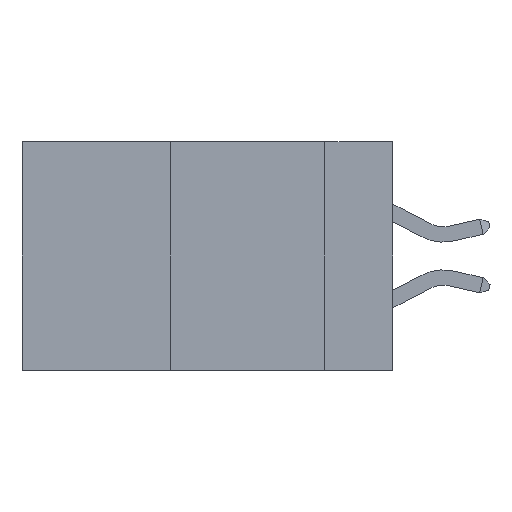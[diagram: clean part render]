
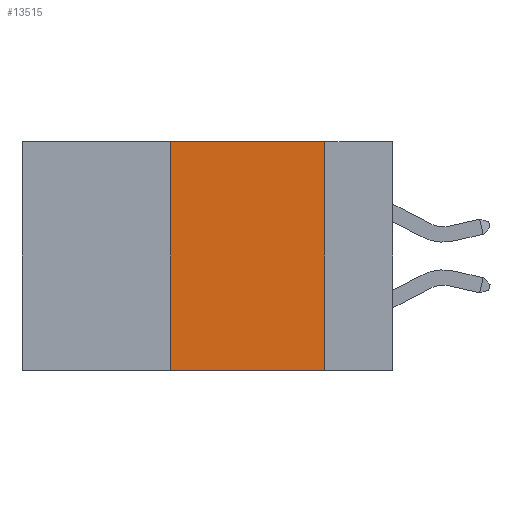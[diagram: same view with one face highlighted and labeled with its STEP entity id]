
A CAD part, left-side view. The second image highlights one B-rep face of the part: STEP entity #13515.
In plain terms, the highlighted planar face has unit normal (-1, 0, 0).
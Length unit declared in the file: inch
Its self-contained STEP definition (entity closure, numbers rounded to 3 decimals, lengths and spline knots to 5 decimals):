
#976 = ORIENTED_EDGE ( 'NONE', *, *, #16483, .F. ) ;
#1418 = LINE ( 'NONE', #15476, #12829 ) ;
#2064 = VECTOR ( 'NONE', #10358, 39.37008 ) ;
#2634 = CARTESIAN_POINT ( 'NONE',  ( 0., 0.11, -0.37 ) ) ;
#2716 = CARTESIAN_POINT ( 'NONE',  ( 0., 0.11, 0. ) ) ;
#6005 = LINE ( 'NONE', #25406, #21736 ) ;
#6934 = EDGE_CURVE ( 'NONE', #15192, #10116, #26371, .T. ) ;
#8670 = VERTEX_POINT ( 'NONE', #2716 ) ;
#9375 = CARTESIAN_POINT ( 'NONE',  ( 0., 0.36, 0. ) ) ;
#10116 = VERTEX_POINT ( 'NONE', #2634 ) ;
#10358 = DIRECTION ( 'NONE',  ( 0., 0., -1. ) ) ;
#12182 = ORIENTED_EDGE ( 'NONE', *, *, #22303, .F. ) ;
#12612 = FACE_OUTER_BOUND ( 'NONE', #16753, .T. ) ;
#12829 = VECTOR ( 'NONE', #30445, 39.37008 ) ;
#13097 = AXIS2_PLACEMENT_3D ( 'NONE', #16803, #19369, #13976 ) ;
#13515 = ADVANCED_FACE ( 'NONE', ( #12612 ), #21570, .F. ) ;
#13782 = DIRECTION ( 'NONE',  ( 0., 0., 1. ) ) ;
#13976 = DIRECTION ( 'NONE',  ( 0., 0., -1. ) ) ;
#15192 = VERTEX_POINT ( 'NONE', #18719 ) ;
#15476 = CARTESIAN_POINT ( 'NONE',  ( 0., 0.6, 0. ) ) ;
#16483 = EDGE_CURVE ( 'NONE', #15192, #19103, #6005, .T. ) ;
#16753 = EDGE_LOOP ( 'NONE', ( #12182, #27725, #976, #28555 ) ) ;
#16803 = CARTESIAN_POINT ( 'NONE',  ( 0., 0.6, 0. ) ) ;
#18719 = CARTESIAN_POINT ( 'NONE',  ( 0., 0.36, -0.37 ) ) ;
#19103 = VERTEX_POINT ( 'NONE', #9375 ) ;
#19369 = DIRECTION ( 'NONE',  ( 1., 0., 0. ) ) ;
#21414 = DIRECTION ( 'NONE',  ( 0., -1., 0. ) ) ;
#21570 = PLANE ( 'NONE',  #13097 ) ;
#21736 = VECTOR ( 'NONE', #13782, 39.37008 ) ;
#21741 = CARTESIAN_POINT ( 'NONE',  ( 0., 0.6, -0.37 ) ) ;
#22303 = EDGE_CURVE ( 'NONE', #8670, #10116, #30381, .T. ) ;
#24787 = VECTOR ( 'NONE', #21414, 39.37008 ) ;
#25406 = CARTESIAN_POINT ( 'NONE',  ( 0., 0.36, 0. ) ) ;
#26371 = LINE ( 'NONE', #21741, #24787 ) ;
#27725 = ORIENTED_EDGE ( 'NONE', *, *, #31428, .F. ) ;
#28555 = ORIENTED_EDGE ( 'NONE', *, *, #6934, .T. ) ;
#30132 = CARTESIAN_POINT ( 'NONE',  ( 0., 0.11, 0. ) ) ;
#30381 = LINE ( 'NONE', #30132, #2064 ) ;
#30445 = DIRECTION ( 'NONE',  ( 0., -1., 0. ) ) ;
#31428 = EDGE_CURVE ( 'NONE', #19103, #8670, #1418, .T. ) ;
